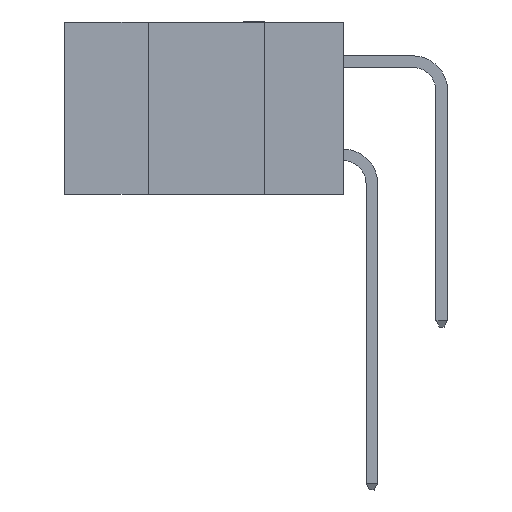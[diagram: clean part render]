
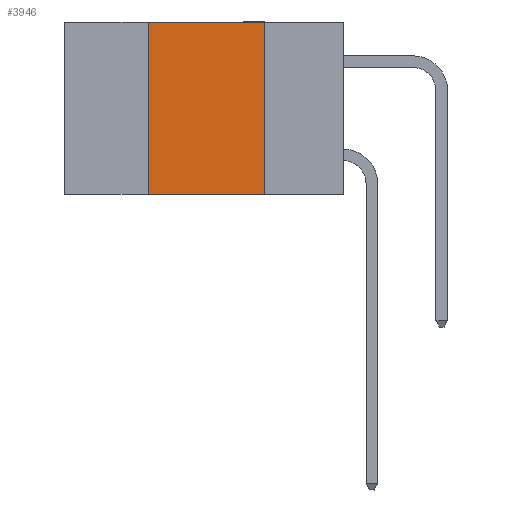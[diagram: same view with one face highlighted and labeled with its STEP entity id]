
A CAD part, left-side view. The second image highlights one B-rep face of the part: STEP entity #3946.
In plain terms, the highlighted planar face has unit normal (-1, 0, 0).
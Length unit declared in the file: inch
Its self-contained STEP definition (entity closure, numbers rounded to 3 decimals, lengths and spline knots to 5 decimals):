
#22 = DIRECTION ( 'NONE',  ( 1., 0., 0. ) ) ;
#194 = EDGE_CURVE ( 'NONE', #8584, #3212, #1239, .T. ) ;
#613 = ORIENTED_EDGE ( 'NONE', *, *, #194, .F. ) ;
#902 = DIRECTION ( 'NONE',  ( 0., -1., 0. ) ) ;
#965 = ORIENTED_EDGE ( 'NONE', *, *, #1240, .F. ) ;
#1239 = LINE ( 'NONE', #9188, #2662 ) ;
#1240 = EDGE_CURVE ( 'NONE', #3212, #11754, #3841, .T. ) ;
#1279 = DIRECTION ( 'NONE',  ( 0., -1., 0. ) ) ;
#1440 = AXIS2_PLACEMENT_3D ( 'NONE', #13384, #22, #13240 ) ;
#1462 = CARTESIAN_POINT ( 'NONE',  ( 0., 0.42, -0.37 ) ) ;
#1709 = VECTOR ( 'NONE', #902, 39.37008 ) ;
#1753 = CARTESIAN_POINT ( 'NONE',  ( 0., 0.6, -0.37 ) ) ;
#1949 = VECTOR ( 'NONE', #6445, 39.37008 ) ;
#2494 = DIRECTION ( 'NONE',  ( 0., 0., 1. ) ) ;
#2662 = VECTOR ( 'NONE', #2494, 39.37008 ) ;
#3212 = VERTEX_POINT ( 'NONE', #5688 ) ;
#3841 = LINE ( 'NONE', #9008, #14282 ) ;
#3946 = ADVANCED_FACE ( 'NONE', ( #10570 ), #5624, .F. ) ;
#3948 = EDGE_CURVE ( 'NONE', #8584, #4524, #4689, .T. ) ;
#4317 = ORIENTED_EDGE ( 'NONE', *, *, #7030, .F. ) ;
#4524 = VERTEX_POINT ( 'NONE', #9494 ) ;
#4689 = LINE ( 'NONE', #1753, #1709 ) ;
#5208 = ORIENTED_EDGE ( 'NONE', *, *, #3948, .T. ) ;
#5624 = PLANE ( 'NONE',  #1440 ) ;
#5688 = CARTESIAN_POINT ( 'NONE',  ( 0., 0.42, 0. ) ) ;
#6445 = DIRECTION ( 'NONE',  ( 0., 0., -1. ) ) ;
#6910 = EDGE_LOOP ( 'NONE', ( #4317, #965, #613, #5208 ) ) ;
#7030 = EDGE_CURVE ( 'NONE', #11754, #4524, #8216, .T. ) ;
#8216 = LINE ( 'NONE', #13028, #1949 ) ;
#8584 = VERTEX_POINT ( 'NONE', #1462 ) ;
#9008 = CARTESIAN_POINT ( 'NONE',  ( 0., 0.6, 0. ) ) ;
#9188 = CARTESIAN_POINT ( 'NONE',  ( 0., 0.42, 0. ) ) ;
#9494 = CARTESIAN_POINT ( 'NONE',  ( 0., 0.17, -0.37 ) ) ;
#10570 = FACE_OUTER_BOUND ( 'NONE', #6910, .T. ) ;
#10744 = CARTESIAN_POINT ( 'NONE',  ( 0., 0.17, 0. ) ) ;
#11754 = VERTEX_POINT ( 'NONE', #10744 ) ;
#13028 = CARTESIAN_POINT ( 'NONE',  ( 0., 0.17, 0. ) ) ;
#13240 = DIRECTION ( 'NONE',  ( 0., 0., -1. ) ) ;
#13384 = CARTESIAN_POINT ( 'NONE',  ( 0., 0.6, 0. ) ) ;
#14282 = VECTOR ( 'NONE', #1279, 39.37008 ) ;
